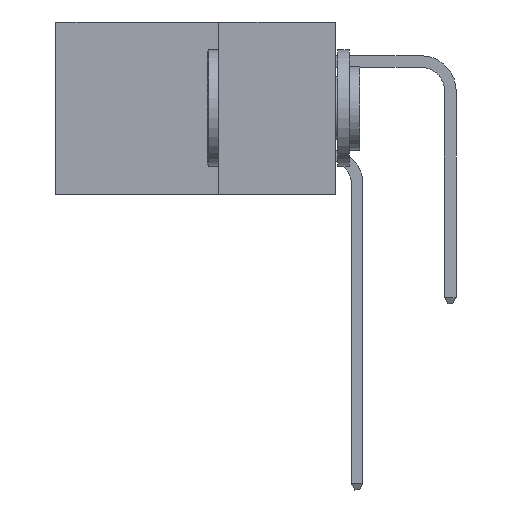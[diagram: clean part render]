
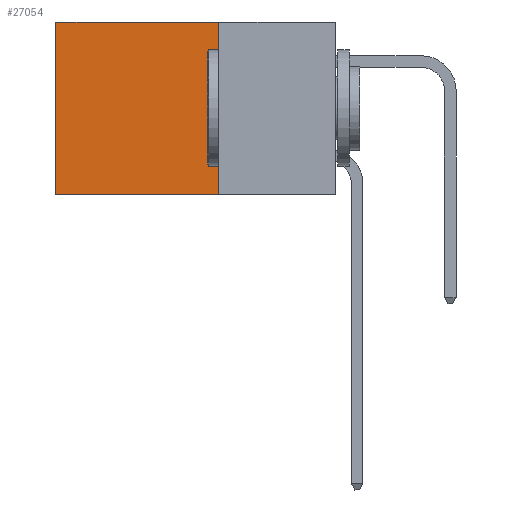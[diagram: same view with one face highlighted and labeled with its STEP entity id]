
A CAD part, left-side view. The second image highlights one B-rep face of the part: STEP entity #27054.
In plain terms, the highlighted planar face has unit normal (-1, 0, 0).
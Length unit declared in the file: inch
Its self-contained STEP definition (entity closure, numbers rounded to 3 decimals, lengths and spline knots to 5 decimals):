
#2828 = PLANE ( 'NONE',  #10468 ) ;
#3679 = CARTESIAN_POINT ( 'NONE',  ( 0.2875, 0.25, 0. ) ) ;
#5830 = CARTESIAN_POINT ( 'NONE',  ( 0.2875, 0.25, 0. ) ) ;
#6842 = EDGE_CURVE ( 'NONE', #26819, #35541, #25196, .T. ) ;
#8318 = CARTESIAN_POINT ( 'NONE',  ( 0.2875, 0.25, -0.37 ) ) ;
#8454 = DIRECTION ( 'NONE',  ( 0., 0., -1. ) ) ;
#8781 = DIRECTION ( 'NONE',  ( 0., 0., -1. ) ) ;
#8904 = ORIENTED_EDGE ( 'NONE', *, *, #6842, .T. ) ;
#9333 = CARTESIAN_POINT ( 'NONE',  ( 0.2875, 0.25, 0. ) ) ;
#9565 = EDGE_CURVE ( 'NONE', #23127, #25641, #19525, .T. ) ;
#10198 = DIRECTION ( 'NONE',  ( 0., 0., -1. ) ) ;
#10468 = AXIS2_PLACEMENT_3D ( 'NONE', #5830, #26551, #8781 ) ;
#11514 = ORIENTED_EDGE ( 'NONE', *, *, #34268, .T. ) ;
#11839 = DIRECTION ( 'NONE',  ( 0., 1., 0. ) ) ;
#13790 = CARTESIAN_POINT ( 'NONE',  ( 0.2875, 0.6, 0. ) ) ;
#17545 = FACE_OUTER_BOUND ( 'NONE', #34990, .T. ) ;
#17827 = LINE ( 'NONE', #8318, #32339 ) ;
#19525 = LINE ( 'NONE', #29136, #33927 ) ;
#23127 = VERTEX_POINT ( 'NONE', #3679 ) ;
#24134 = CARTESIAN_POINT ( 'NONE',  ( 0.2875, 0.25, -0.37 ) ) ;
#25196 = LINE ( 'NONE', #30676, #31964 ) ;
#25641 = VERTEX_POINT ( 'NONE', #24134 ) ;
#26251 = ORIENTED_EDGE ( 'NONE', *, *, #9565, .F. ) ;
#26551 = DIRECTION ( 'NONE',  ( 1., 0., 0. ) ) ;
#26819 = VERTEX_POINT ( 'NONE', #13790 ) ;
#27054 = ADVANCED_FACE ( 'NONE', ( #17545 ), #2828, .F. ) ;
#29034 = EDGE_CURVE ( 'NONE', #25641, #35541, #17827, .T. ) ;
#29136 = CARTESIAN_POINT ( 'NONE',  ( 0.2875, 0.25, 0. ) ) ;
#29711 = CARTESIAN_POINT ( 'NONE',  ( 0.2875, 0.6, -0.37 ) ) ;
#30676 = CARTESIAN_POINT ( 'NONE',  ( 0.2875, 0.6, 0. ) ) ;
#30722 = VECTOR ( 'NONE', #32808, 39.37008 ) ;
#31634 = LINE ( 'NONE', #9333, #30722 ) ;
#31964 = VECTOR ( 'NONE', #10198, 39.37008 ) ;
#32339 = VECTOR ( 'NONE', #11839, 39.37008 ) ;
#32808 = DIRECTION ( 'NONE',  ( 0., 1., 0. ) ) ;
#33927 = VECTOR ( 'NONE', #8454, 39.37008 ) ;
#34268 = EDGE_CURVE ( 'NONE', #23127, #26819, #31634, .T. ) ;
#34990 = EDGE_LOOP ( 'NONE', ( #8904, #37808, #26251, #11514 ) ) ;
#35541 = VERTEX_POINT ( 'NONE', #29711 ) ;
#37808 = ORIENTED_EDGE ( 'NONE', *, *, #29034, .F. ) ;
